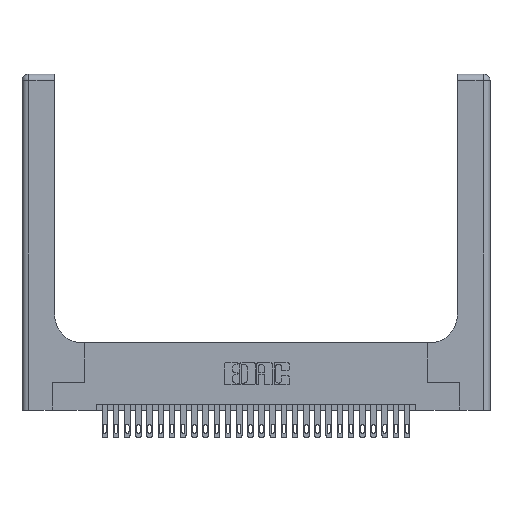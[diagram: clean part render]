
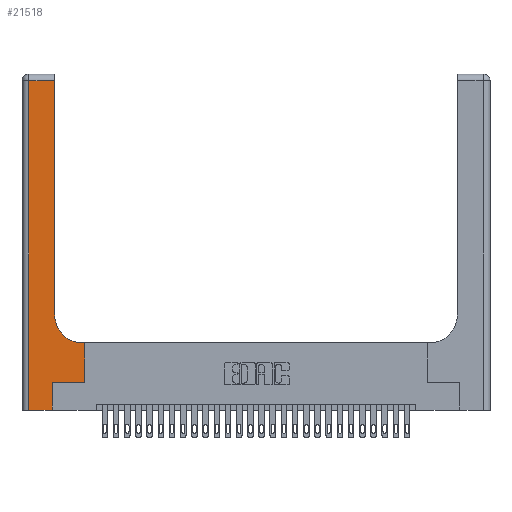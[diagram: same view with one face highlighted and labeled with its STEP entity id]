
A CAD part, top view. The second image highlights one B-rep face of the part: STEP entity #21518.
In plain terms, the highlighted planar face has unit normal (0, 0, 1).
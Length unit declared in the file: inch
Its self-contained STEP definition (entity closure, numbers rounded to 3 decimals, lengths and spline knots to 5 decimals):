
#788 = ORIENTED_EDGE ( 'NONE', *, *, #27107, .T. ) ;
#1189 = CARTESIAN_POINT ( 'NONE',  ( 0.269, 0., 0.37 ) ) ;
#1206 = DIRECTION ( 'NONE',  ( 0., -1., 0. ) ) ;
#1298 = CARTESIAN_POINT ( 'NONE',  ( 0.06, 2.94, 0.37 ) ) ;
#1431 = LINE ( 'NONE', #23502, #21048 ) ;
#1956 = DIRECTION ( 'NONE',  ( -1., 0., 0. ) ) ;
#2486 = VERTEX_POINT ( 'NONE', #25691 ) ;
#2674 = ORIENTED_EDGE ( 'NONE', *, *, #17371, .T. ) ;
#5359 = ORIENTED_EDGE ( 'NONE', *, *, #10343, .T. ) ;
#5958 = VERTEX_POINT ( 'NONE', #24845 ) ;
#6062 = CARTESIAN_POINT ( 'NONE',  ( 0.2915, 3., 0.37 ) ) ;
#6122 = EDGE_CURVE ( 'NONE', #12922, #6700, #17731, .T. ) ;
#6259 = EDGE_LOOP ( 'NONE', ( #10211, #23754, #19187, #788, #5359, #23374, #13528, #12871, #2674 ) ) ;
#6700 = VERTEX_POINT ( 'NONE', #26217 ) ;
#7096 = DIRECTION ( 'NONE',  ( 0., 1., 0. ) ) ;
#7806 = CARTESIAN_POINT ( 'NONE',  ( 0.5415, 0.85, 0.37 ) ) ;
#8789 = DIRECTION ( 'NONE',  ( 1., 0., 0. ) ) ;
#9106 = FACE_OUTER_BOUND ( 'NONE', #6259, .T. ) ;
#9747 = VECTOR ( 'NONE', #8789, 39.37008 ) ;
#9862 = EDGE_CURVE ( 'NONE', #6700, #18810, #1431, .T. ) ;
#10060 = DIRECTION ( 'NONE',  ( 1., 0., 0. ) ) ;
#10211 = ORIENTED_EDGE ( 'NONE', *, *, #14146, .T. ) ;
#10343 = EDGE_CURVE ( 'NONE', #15690, #5958, #12211, .T. ) ;
#11858 = CARTESIAN_POINT ( 'NONE',  ( 0.5585, 0.25, 0.37 ) ) ;
#12138 = PLANE ( 'NONE',  #28925 ) ;
#12211 = LINE ( 'NONE', #13488, #25530 ) ;
#12835 = LINE ( 'NONE', #23255, #13164 ) ;
#12871 = ORIENTED_EDGE ( 'NONE', *, *, #9862, .T. ) ;
#12922 = VERTEX_POINT ( 'NONE', #27930 ) ;
#13164 = VECTOR ( 'NONE', #27756, 39.37008 ) ;
#13488 = CARTESIAN_POINT ( 'NONE',  ( 0.269, 0., 0.37 ) ) ;
#13528 = ORIENTED_EDGE ( 'NONE', *, *, #6122, .T. ) ;
#13619 = DIRECTION ( 'NONE',  ( 1., 0., 0. ) ) ;
#13800 = EDGE_CURVE ( 'NONE', #21578, #21957, #22444, .T. ) ;
#13912 = VECTOR ( 'NONE', #13619, 39.37008 ) ;
#14146 = EDGE_CURVE ( 'NONE', #2486, #28502, #19277, .T. ) ;
#14575 = CIRCLE ( 'NONE', #24011, 0.25 ) ;
#14835 = DIRECTION ( 'NONE',  ( 0., 1., 0. ) ) ;
#15690 = VERTEX_POINT ( 'NONE', #1189 ) ;
#15824 = CARTESIAN_POINT ( 'NONE',  ( 0.06, 0., 0.37 ) ) ;
#16952 = DIRECTION ( 'NONE',  ( 0., 0., -1. ) ) ;
#17371 = EDGE_CURVE ( 'NONE', #18810, #2486, #14575, .T. ) ;
#17731 = LINE ( 'NONE', #11858, #26818 ) ;
#18113 = CARTESIAN_POINT ( 'NONE',  ( 0.2915, 2.94, 0.37 ) ) ;
#18810 = VERTEX_POINT ( 'NONE', #26189 ) ;
#18854 = LINE ( 'NONE', #22354, #13912 ) ;
#19187 = ORIENTED_EDGE ( 'NONE', *, *, #13800, .T. ) ;
#19277 = LINE ( 'NONE', #6062, #24196 ) ;
#20434 = CARTESIAN_POINT ( 'NONE',  ( 0.06, 3., 0.37 ) ) ;
#21048 = VECTOR ( 'NONE', #1956, 39.37008 ) ;
#21359 = CARTESIAN_POINT ( 'NONE',  ( 0., 3., 0.37 ) ) ;
#21406 = VECTOR ( 'NONE', #1206, 39.37008 ) ;
#21518 = ADVANCED_FACE ( 'NONE', ( #9106 ), #12138, .F. ) ;
#21578 = VERTEX_POINT ( 'NONE', #1298 ) ;
#21957 = VERTEX_POINT ( 'NONE', #15824 ) ;
#22229 = CARTESIAN_POINT ( 'NONE',  ( 0., 0., 0.37 ) ) ;
#22354 = CARTESIAN_POINT ( 'NONE',  ( 0.269, 0.25, 0.37 ) ) ;
#22444 = LINE ( 'NONE', #20434, #21406 ) ;
#23255 = CARTESIAN_POINT ( 'NONE',  ( 0., 2.94, 0.37 ) ) ;
#23374 = ORIENTED_EDGE ( 'NONE', *, *, #28469, .T. ) ;
#23501 = DIRECTION ( 'NONE',  ( 0., 0., -1. ) ) ;
#23502 = CARTESIAN_POINT ( 'NONE',  ( 0.2915, 0.6, 0.37 ) ) ;
#23754 = ORIENTED_EDGE ( 'NONE', *, *, #24944, .T. ) ;
#24011 = AXIS2_PLACEMENT_3D ( 'NONE', #7806, #23501, #10060 ) ;
#24196 = VECTOR ( 'NONE', #26206, 39.37008 ) ;
#24845 = CARTESIAN_POINT ( 'NONE',  ( 0.269, 0.25, 0.37 ) ) ;
#24944 = EDGE_CURVE ( 'NONE', #28502, #21578, #12835, .T. ) ;
#25530 = VECTOR ( 'NONE', #7096, 39.37008 ) ;
#25691 = CARTESIAN_POINT ( 'NONE',  ( 0.2915, 0.85, 0.37 ) ) ;
#25947 = DIRECTION ( 'NONE',  ( -1., 0., 0. ) ) ;
#26189 = CARTESIAN_POINT ( 'NONE',  ( 0.5415, 0.6, 0.37 ) ) ;
#26206 = DIRECTION ( 'NONE',  ( 0., 1., 0. ) ) ;
#26217 = CARTESIAN_POINT ( 'NONE',  ( 0.5585, 0.6, 0.37 ) ) ;
#26818 = VECTOR ( 'NONE', #14835, 39.37008 ) ;
#27107 = EDGE_CURVE ( 'NONE', #21957, #15690, #27635, .T. ) ;
#27635 = LINE ( 'NONE', #22229, #9747 ) ;
#27756 = DIRECTION ( 'NONE',  ( -1., 0., 0. ) ) ;
#27930 = CARTESIAN_POINT ( 'NONE',  ( 0.5585, 0.25, 0.37 ) ) ;
#28469 = EDGE_CURVE ( 'NONE', #5958, #12922, #18854, .T. ) ;
#28502 = VERTEX_POINT ( 'NONE', #18113 ) ;
#28925 = AXIS2_PLACEMENT_3D ( 'NONE', #21359, #16952, #25947 ) ;
